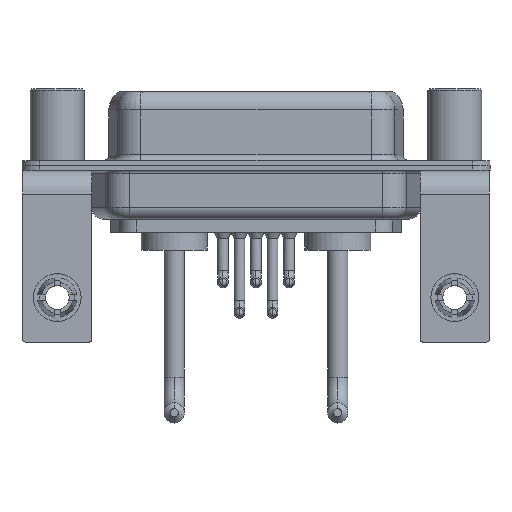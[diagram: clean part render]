
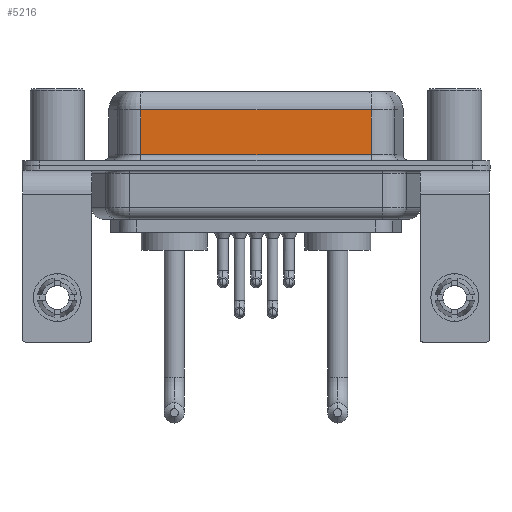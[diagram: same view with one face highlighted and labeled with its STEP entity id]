
A CAD part, front view. The second image highlights one B-rep face of the part: STEP entity #5216.
In plain terms, the highlighted planar face has unit normal (0, -1, 0).
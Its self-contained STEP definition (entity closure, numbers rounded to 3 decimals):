
#88 = LINE ( 'NONE', #5095, #2355 ) ;
#929 = EDGE_CURVE ( 'NONE', #14461, #15025, #17376, .T. ) ;
#2355 = VECTOR ( 'NONE', #11480, 1000. ) ;
#4159 = VECTOR ( 'NONE', #6057, 1000. ) ;
#4456 = VERTEX_POINT ( 'NONE', #8779 ) ;
#4646 = CARTESIAN_POINT ( 'NONE',  ( 26.287, -3.95, 4.65 ) ) ;
#4848 = CARTESIAN_POINT ( 'NONE',  ( 7.013, -3.95, 0.9 ) ) ;
#4925 = EDGE_LOOP ( 'NONE', ( #15580, #10373, #7251, #11377 ) ) ;
#4983 = CARTESIAN_POINT ( 'NONE',  ( 26.287, -3.95, 6.4 ) ) ;
#5095 = CARTESIAN_POINT ( 'NONE',  ( 26.287, -3.95, 0.9 ) ) ;
#5178 = DIRECTION ( 'NONE',  ( 0., 0., 1. ) ) ;
#5208 = DIRECTION ( 'NONE',  ( 0., 0., -1. ) ) ;
#5216 = ADVANCED_FACE ( 'NONE', ( #16575 ), #6782, .F. ) ;
#6057 = DIRECTION ( 'NONE',  ( -1., 0., 0. ) ) ;
#6492 = LINE ( 'NONE', #4983, #19249 ) ;
#6564 = EDGE_CURVE ( 'NONE', #4456, #16803, #6492, .T. ) ;
#6782 = PLANE ( 'NONE',  #15695 ) ;
#7251 = ORIENTED_EDGE ( 'NONE', *, *, #929, .T. ) ;
#7447 = LINE ( 'NONE', #4646, #4159 ) ;
#8169 = EDGE_CURVE ( 'NONE', #4456, #14461, #7447, .T. ) ;
#8779 = CARTESIAN_POINT ( 'NONE',  ( 26.287, -3.95, 4.65 ) ) ;
#10373 = ORIENTED_EDGE ( 'NONE', *, *, #8169, .T. ) ;
#11262 = CARTESIAN_POINT ( 'NONE',  ( 7.013, -3.95, 4.65 ) ) ;
#11268 = CARTESIAN_POINT ( 'NONE',  ( 26.287, -3.95, 0.9 ) ) ;
#11377 = ORIENTED_EDGE ( 'NONE', *, *, #18335, .T. ) ;
#11480 = DIRECTION ( 'NONE',  ( 1., 0., 0. ) ) ;
#12476 = DIRECTION ( 'NONE',  ( 0., 0., -1. ) ) ;
#14461 = VERTEX_POINT ( 'NONE', #11262 ) ;
#15025 = VERTEX_POINT ( 'NONE', #4848 ) ;
#15113 = DIRECTION ( 'NONE',  ( 0., 1., 0. ) ) ;
#15580 = ORIENTED_EDGE ( 'NONE', *, *, #6564, .F. ) ;
#15695 = AXIS2_PLACEMENT_3D ( 'NONE', #18394, #15113, #5178 ) ;
#16575 = FACE_OUTER_BOUND ( 'NONE', #4925, .T. ) ;
#16803 = VERTEX_POINT ( 'NONE', #11268 ) ;
#17376 = LINE ( 'NONE', #17472, #21005 ) ;
#17472 = CARTESIAN_POINT ( 'NONE',  ( 7.013, -3.95, 6.4 ) ) ;
#18335 = EDGE_CURVE ( 'NONE', #15025, #16803, #88, .T. ) ;
#18394 = CARTESIAN_POINT ( 'NONE',  ( 26.287, -3.95, 6.4 ) ) ;
#19249 = VECTOR ( 'NONE', #5208, 1000. ) ;
#21005 = VECTOR ( 'NONE', #12476, 1000. ) ;
